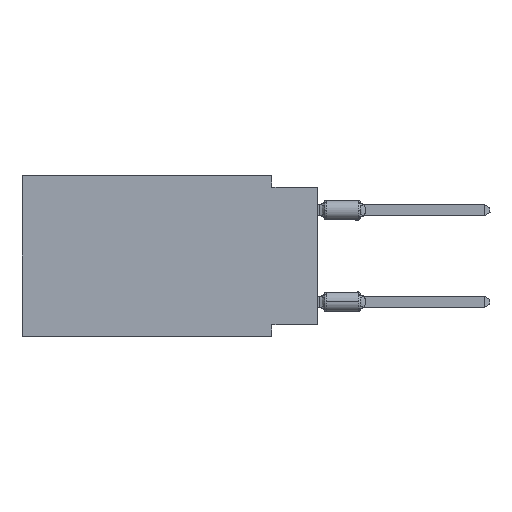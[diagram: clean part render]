
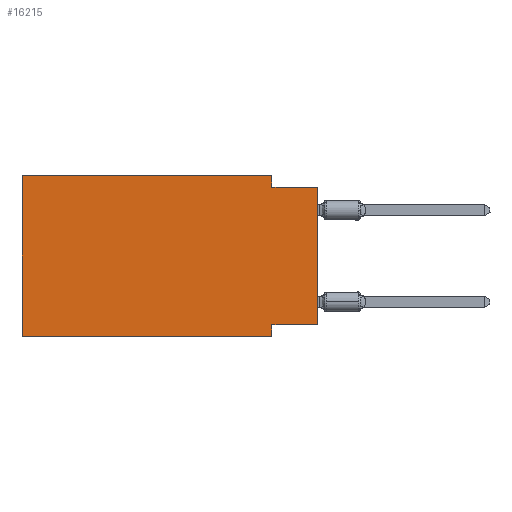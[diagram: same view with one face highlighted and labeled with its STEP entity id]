
A CAD part, left-side view. The second image highlights one B-rep face of the part: STEP entity #16215.
In plain terms, the highlighted planar face has unit normal (-1, 0, 0).
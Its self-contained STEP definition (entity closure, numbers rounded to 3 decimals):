
#2 = CARTESIAN_POINT ( 'NONE',  ( 0., 16.383, 0. ) ) ;
#74 = EDGE_CURVE ( 'NONE', #17448, #15852, #62208, .T. ) ;
#968 = VECTOR ( 'NONE', #33120, 1000. ) ;
#969 = VECTOR ( 'NONE', #28932, 1000. ) ;
#3165 = VECTOR ( 'NONE', #22683, 1000. ) ;
#3919 = CARTESIAN_POINT ( 'NONE',  ( 0., 2.54, 0. ) ) ;
#5526 = CARTESIAN_POINT ( 'NONE',  ( 0., 0., -8.255 ) ) ;
#6700 = LINE ( 'NONE', #64437, #25289 ) ;
#8965 = DIRECTION ( 'NONE',  ( 0., 0., -1. ) ) ;
#9340 = CARTESIAN_POINT ( 'NONE',  ( 0., 2.54, 0. ) ) ;
#9819 = VERTEX_POINT ( 'NONE', #49014 ) ;
#12137 = CARTESIAN_POINT ( 'NONE',  ( 0., 2.54, -8.255 ) ) ;
#13482 = VECTOR ( 'NONE', #45478, 1000. ) ;
#14513 = CARTESIAN_POINT ( 'NONE',  ( 0., 16.383, -8.89 ) ) ;
#15304 = CARTESIAN_POINT ( 'NONE',  ( 0., 16.383, 0. ) ) ;
#15852 = VERTEX_POINT ( 'NONE', #3919 ) ;
#16215 = ADVANCED_FACE ( 'NONE', ( #71186 ), #20163, .F. ) ;
#17448 = VERTEX_POINT ( 'NONE', #17959 ) ;
#17577 = EDGE_CURVE ( 'NONE', #65386, #33275, #70105, .T. ) ;
#17959 = CARTESIAN_POINT ( 'NONE',  ( 0., 16.383, 0. ) ) ;
#19350 = AXIS2_PLACEMENT_3D ( 'NONE', #15304, #60014, #8965 ) ;
#20163 = PLANE ( 'NONE',  #19350 ) ;
#21182 = LINE ( 'NONE', #14513, #57679 ) ;
#21260 = DIRECTION ( 'NONE',  ( 0., 0., -1. ) ) ;
#21268 = EDGE_LOOP ( 'NONE', ( #28215, #55659, #55848, #48666, #45069, #40966, #35531, #32320 ) ) ;
#22683 = DIRECTION ( 'NONE',  ( 0., 1., 0. ) ) ;
#25289 = VECTOR ( 'NONE', #35794, 1000. ) ;
#26357 = EDGE_CURVE ( 'NONE', #38644, #69627, #63538, .T. ) ;
#28117 = CARTESIAN_POINT ( 'NONE',  ( 0., 2.54, -8.89 ) ) ;
#28215 = ORIENTED_EDGE ( 'NONE', *, *, #26357, .T. ) ;
#28932 = DIRECTION ( 'NONE',  ( 0., 0., 1. ) ) ;
#29466 = CARTESIAN_POINT ( 'NONE',  ( 0., 0., -0.635 ) ) ;
#32320 = ORIENTED_EDGE ( 'NONE', *, *, #37878, .F. ) ;
#33120 = DIRECTION ( 'NONE',  ( 0., -1., 0. ) ) ;
#33275 = VERTEX_POINT ( 'NONE', #28117 ) ;
#33880 = LINE ( 'NONE', #5526, #3165 ) ;
#35531 = ORIENTED_EDGE ( 'NONE', *, *, #17577, .F. ) ;
#35794 = DIRECTION ( 'NONE',  ( 0., 0., 1. ) ) ;
#36397 = EDGE_CURVE ( 'NONE', #9819, #33275, #21182, .T. ) ;
#37341 = CARTESIAN_POINT ( 'NONE',  ( 0., 2.54, -0.635 ) ) ;
#37878 = EDGE_CURVE ( 'NONE', #38644, #65386, #33880, .T. ) ;
#38644 = VERTEX_POINT ( 'NONE', #65187 ) ;
#40966 = ORIENTED_EDGE ( 'NONE', *, *, #36397, .T. ) ;
#43579 = LINE ( 'NONE', #66242, #968 ) ;
#43767 = EDGE_CURVE ( 'NONE', #59946, #69627, #43579, .T. ) ;
#44069 = EDGE_CURVE ( 'NONE', #15852, #59946, #60745, .T. ) ;
#45069 = ORIENTED_EDGE ( 'NONE', *, *, #69596, .F. ) ;
#45478 = DIRECTION ( 'NONE',  ( 0., -1., 0. ) ) ;
#46067 = CARTESIAN_POINT ( 'NONE',  ( 0., 0., 0. ) ) ;
#48591 = VECTOR ( 'NONE', #21260, 1000. ) ;
#48666 = ORIENTED_EDGE ( 'NONE', *, *, #74, .F. ) ;
#49014 = CARTESIAN_POINT ( 'NONE',  ( 0., 16.383, -8.89 ) ) ;
#53714 = DIRECTION ( 'NONE',  ( 0., 0., -1. ) ) ;
#55659 = ORIENTED_EDGE ( 'NONE', *, *, #43767, .F. ) ;
#55848 = ORIENTED_EDGE ( 'NONE', *, *, #44069, .F. ) ;
#57679 = VECTOR ( 'NONE', #60672, 1000. ) ;
#59946 = VERTEX_POINT ( 'NONE', #37341 ) ;
#60014 = DIRECTION ( 'NONE',  ( 1., 0., 0. ) ) ;
#60021 = CARTESIAN_POINT ( 'NONE',  ( 0., 2.54, -8.89 ) ) ;
#60672 = DIRECTION ( 'NONE',  ( 0., -1., 0. ) ) ;
#60745 = LINE ( 'NONE', #9340, #48591 ) ;
#61140 = VECTOR ( 'NONE', #53714, 1000. ) ;
#62208 = LINE ( 'NONE', #2, #13482 ) ;
#63538 = LINE ( 'NONE', #46067, #969 ) ;
#64437 = CARTESIAN_POINT ( 'NONE',  ( 0., 16.383, 0. ) ) ;
#65187 = CARTESIAN_POINT ( 'NONE',  ( 0., 0., -8.255 ) ) ;
#65386 = VERTEX_POINT ( 'NONE', #12137 ) ;
#66242 = CARTESIAN_POINT ( 'NONE',  ( 0., 0., -0.635 ) ) ;
#69596 = EDGE_CURVE ( 'NONE', #9819, #17448, #6700, .T. ) ;
#69627 = VERTEX_POINT ( 'NONE', #29466 ) ;
#70105 = LINE ( 'NONE', #60021, #61140 ) ;
#71186 = FACE_OUTER_BOUND ( 'NONE', #21268, .T. ) ;
